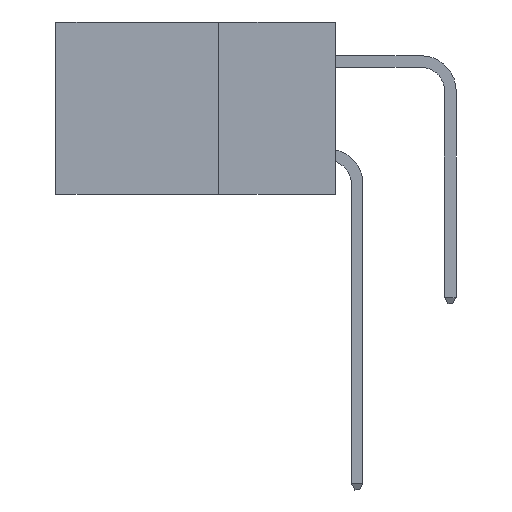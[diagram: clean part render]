
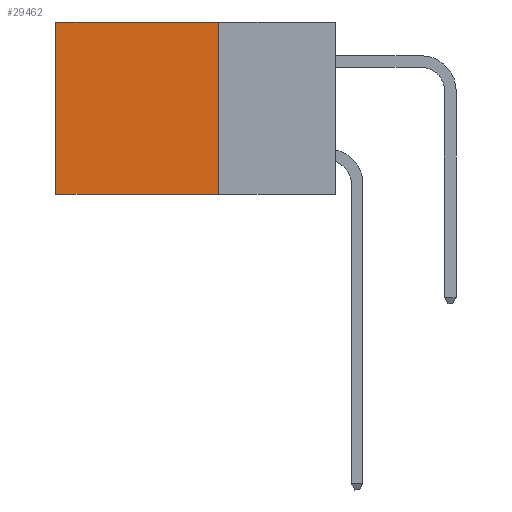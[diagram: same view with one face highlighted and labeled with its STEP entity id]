
A CAD part, left-side view. The second image highlights one B-rep face of the part: STEP entity #29462.
In plain terms, the highlighted planar face has unit normal (-1, 0, 0).
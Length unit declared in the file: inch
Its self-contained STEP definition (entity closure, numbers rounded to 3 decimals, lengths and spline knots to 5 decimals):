
#2421 = EDGE_CURVE ( 'NONE', #32391, #14309, #38477, .T. ) ;
#3852 = VECTOR ( 'NONE', #23421, 39.37008 ) ;
#4115 = AXIS2_PLACEMENT_3D ( 'NONE', #7527, #28722, #16384 ) ;
#4459 = PLANE ( 'NONE',  #4115 ) ;
#6182 = CARTESIAN_POINT ( 'NONE',  ( 0.2875, 0.6, 0. ) ) ;
#7527 = CARTESIAN_POINT ( 'NONE',  ( 0.2875, 0.25, 0. ) ) ;
#7572 = ORIENTED_EDGE ( 'NONE', *, *, #17427, .T. ) ;
#9210 = VERTEX_POINT ( 'NONE', #32510 ) ;
#11739 = ORIENTED_EDGE ( 'NONE', *, *, #30160, .F. ) ;
#11872 = CARTESIAN_POINT ( 'NONE',  ( 0.2875, 0.25, 0. ) ) ;
#13275 = FACE_OUTER_BOUND ( 'NONE', #20477, .T. ) ;
#14017 = CARTESIAN_POINT ( 'NONE',  ( 0.2875, 0.25, 0. ) ) ;
#14309 = VERTEX_POINT ( 'NONE', #22977 ) ;
#14529 = DIRECTION ( 'NONE',  ( 0., 1., 0. ) ) ;
#16384 = DIRECTION ( 'NONE',  ( 0., 0., -1. ) ) ;
#17364 = ORIENTED_EDGE ( 'NONE', *, *, #35213, .T. ) ;
#17427 = EDGE_CURVE ( 'NONE', #32391, #29196, #31301, .T. ) ;
#20477 = EDGE_LOOP ( 'NONE', ( #17364, #11739, #34529, #7572 ) ) ;
#22774 = VECTOR ( 'NONE', #14529, 39.37008 ) ;
#22977 = CARTESIAN_POINT ( 'NONE',  ( 0.2875, 0.25, -0.37 ) ) ;
#23421 = DIRECTION ( 'NONE',  ( 0., 0., -1. ) ) ;
#25463 = DIRECTION ( 'NONE',  ( 0., 1., 0. ) ) ;
#25942 = CARTESIAN_POINT ( 'NONE',  ( 0.2875, 0.6, 0. ) ) ;
#28722 = DIRECTION ( 'NONE',  ( 1., 0., 0. ) ) ;
#28803 = CARTESIAN_POINT ( 'NONE',  ( 0.2875, 0.25, -0.37 ) ) ;
#29196 = VERTEX_POINT ( 'NONE', #6182 ) ;
#29462 = ADVANCED_FACE ( 'NONE', ( #13275 ), #4459, .F. ) ;
#30160 = EDGE_CURVE ( 'NONE', #14309, #9210, #38931, .T. ) ;
#31301 = LINE ( 'NONE', #37652, #22774 ) ;
#31675 = DIRECTION ( 'NONE',  ( 0., 0., -1. ) ) ;
#32391 = VERTEX_POINT ( 'NONE', #14017 ) ;
#32510 = CARTESIAN_POINT ( 'NONE',  ( 0.2875, 0.6, -0.37 ) ) ;
#34529 = ORIENTED_EDGE ( 'NONE', *, *, #2421, .F. ) ;
#35213 = EDGE_CURVE ( 'NONE', #29196, #9210, #35798, .T. ) ;
#35798 = LINE ( 'NONE', #25942, #38151 ) ;
#36560 = VECTOR ( 'NONE', #25463, 39.37008 ) ;
#37652 = CARTESIAN_POINT ( 'NONE',  ( 0.2875, 0.25, 0. ) ) ;
#38151 = VECTOR ( 'NONE', #31675, 39.37008 ) ;
#38477 = LINE ( 'NONE', #11872, #3852 ) ;
#38931 = LINE ( 'NONE', #28803, #36560 ) ;
